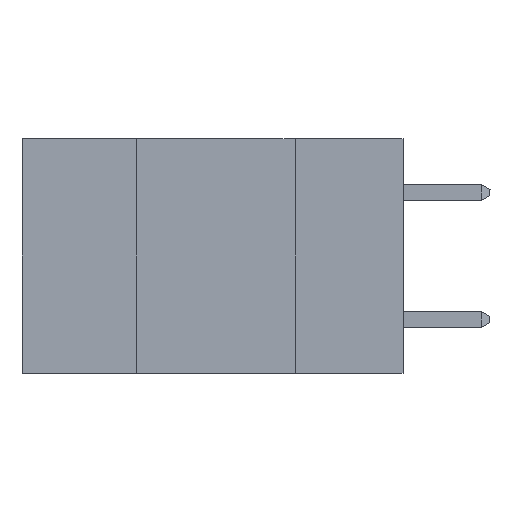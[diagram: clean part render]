
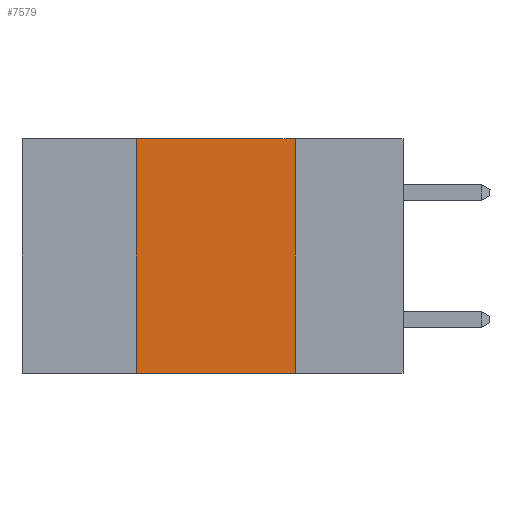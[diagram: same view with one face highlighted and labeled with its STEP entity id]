
A CAD part, left-side view. The second image highlights one B-rep face of the part: STEP entity #7579.
In plain terms, the highlighted planar face has unit normal (-1, 0, 0).
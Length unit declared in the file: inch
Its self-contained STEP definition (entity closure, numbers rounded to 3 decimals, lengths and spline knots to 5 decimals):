
#1066 = EDGE_CURVE ( 'NONE', #6474, #18505, #1148, .T. ) ;
#1148 = LINE ( 'NONE', #2206, #17209 ) ;
#2206 = CARTESIAN_POINT ( 'NONE',  ( 0., 0.6, -0.37 ) ) ;
#2532 = VECTOR ( 'NONE', #18466, 39.37008 ) ;
#4163 = AXIS2_PLACEMENT_3D ( 'NONE', #17145, #18750, #8898 ) ;
#4492 = CARTESIAN_POINT ( 'NONE',  ( 0., 0.17, 0. ) ) ;
#4827 = ORIENTED_EDGE ( 'NONE', *, *, #18640, .F. ) ;
#4903 = VERTEX_POINT ( 'NONE', #13752 ) ;
#5522 = PLANE ( 'NONE',  #4163 ) ;
#6474 = VERTEX_POINT ( 'NONE', #20088 ) ;
#6916 = CARTESIAN_POINT ( 'NONE',  ( 0., 0.42, 0. ) ) ;
#7579 = ADVANCED_FACE ( 'NONE', ( #20663 ), #5522, .F. ) ;
#8898 = DIRECTION ( 'NONE',  ( 0., 0., -1. ) ) ;
#9798 = ORIENTED_EDGE ( 'NONE', *, *, #17110, .F. ) ;
#10488 = CARTESIAN_POINT ( 'NONE',  ( 0., 0.42, 0. ) ) ;
#10664 = DIRECTION ( 'NONE',  ( 0., -1., 0. ) ) ;
#11110 = LINE ( 'NONE', #6916, #2532 ) ;
#12321 = LINE ( 'NONE', #17258, #20355 ) ;
#12815 = EDGE_CURVE ( 'NONE', #4903, #18505, #14684, .T. ) ;
#13584 = DIRECTION ( 'NONE',  ( 0., -1., 0. ) ) ;
#13752 = CARTESIAN_POINT ( 'NONE',  ( 0., 0.17, 0. ) ) ;
#14684 = LINE ( 'NONE', #4492, #18306 ) ;
#15386 = VERTEX_POINT ( 'NONE', #10488 ) ;
#15568 = EDGE_LOOP ( 'NONE', ( #20745, #4827, #9798, #17419 ) ) ;
#17110 = EDGE_CURVE ( 'NONE', #6474, #15386, #11110, .T. ) ;
#17145 = CARTESIAN_POINT ( 'NONE',  ( 0., 0.6, 0. ) ) ;
#17209 = VECTOR ( 'NONE', #13584, 39.37008 ) ;
#17258 = CARTESIAN_POINT ( 'NONE',  ( 0., 0.6, 0. ) ) ;
#17419 = ORIENTED_EDGE ( 'NONE', *, *, #1066, .T. ) ;
#18306 = VECTOR ( 'NONE', #18577, 39.37008 ) ;
#18421 = CARTESIAN_POINT ( 'NONE',  ( 0., 0.17, -0.37 ) ) ;
#18466 = DIRECTION ( 'NONE',  ( 0., 0., 1. ) ) ;
#18505 = VERTEX_POINT ( 'NONE', #18421 ) ;
#18577 = DIRECTION ( 'NONE',  ( 0., 0., -1. ) ) ;
#18640 = EDGE_CURVE ( 'NONE', #15386, #4903, #12321, .T. ) ;
#18750 = DIRECTION ( 'NONE',  ( 1., 0., 0. ) ) ;
#20088 = CARTESIAN_POINT ( 'NONE',  ( 0., 0.42, -0.37 ) ) ;
#20355 = VECTOR ( 'NONE', #10664, 39.37008 ) ;
#20663 = FACE_OUTER_BOUND ( 'NONE', #15568, .T. ) ;
#20745 = ORIENTED_EDGE ( 'NONE', *, *, #12815, .F. ) ;
